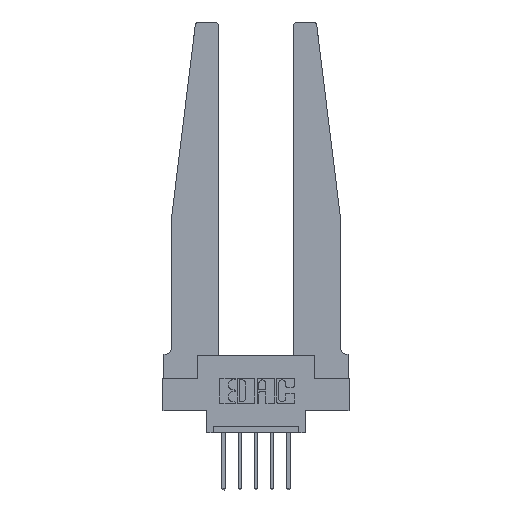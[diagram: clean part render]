
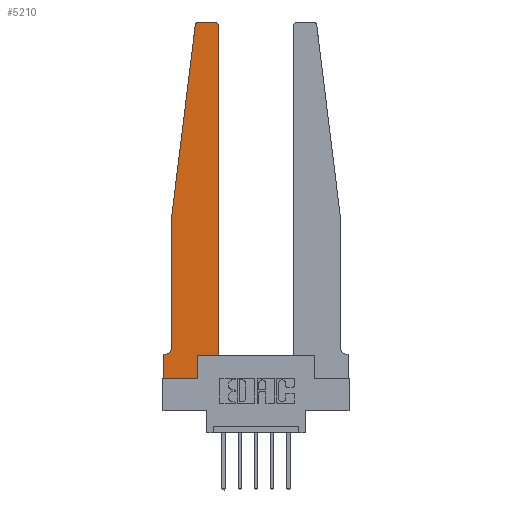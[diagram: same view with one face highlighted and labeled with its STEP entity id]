
A CAD part, top view. The second image highlights one B-rep face of the part: STEP entity #5210.
In plain terms, the highlighted planar face has unit normal (0, 0, 1).
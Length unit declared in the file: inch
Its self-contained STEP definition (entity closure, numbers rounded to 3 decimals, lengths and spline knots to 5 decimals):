
#15 = ORIENTED_EDGE ( 'NONE', *, *, #7606, .T. ) ;
#310 = CARTESIAN_POINT ( 'NONE',  ( 0., 0., 0.37 ) ) ;
#470 = CARTESIAN_POINT ( 'NONE',  ( 0.065, 1.25, 0.37 ) ) ;
#858 = ORIENTED_EDGE ( 'NONE', *, *, #10404, .T. ) ;
#1111 = VERTEX_POINT ( 'NONE', #8150 ) ;
#1137 = LINE ( 'NONE', #5262, #3582 ) ;
#1139 = LINE ( 'NONE', #310, #9951 ) ;
#1143 = ORIENTED_EDGE ( 'NONE', *, *, #5198, .T. ) ;
#1299 = VECTOR ( 'NONE', #4682, 39.37008 ) ;
#1489 = CARTESIAN_POINT ( 'NONE',  ( 0.2605, 0., 0.37 ) ) ;
#1710 = VECTOR ( 'NONE', #10399, 39.37008 ) ;
#1847 = LINE ( 'NONE', #5696, #1299 ) ;
#2155 = LINE ( 'NONE', #5459, #3050 ) ;
#2322 = CARTESIAN_POINT ( 'NONE',  ( 0.065, 0.2375, 0.37 ) ) ;
#2347 = CARTESIAN_POINT ( 'NONE',  ( 0.015, 0.1875, 0.37 ) ) ;
#2419 = DIRECTION ( 'NONE',  ( 0., 0., 1. ) ) ;
#2442 = ORIENTED_EDGE ( 'NONE', *, *, #10796, .T. ) ;
#2529 = AXIS2_PLACEMENT_3D ( 'NONE', #10632, #11456, #9399 ) ;
#2594 = DIRECTION ( 'NONE',  ( 0., 0., 1. ) ) ;
#2782 = DIRECTION ( 'NONE',  ( -0.122, -0.992, 0. ) ) ;
#2896 = EDGE_CURVE ( 'NONE', #4241, #7822, #4874, .T. ) ;
#3050 = VECTOR ( 'NONE', #6332, 39.37008 ) ;
#3070 = DIRECTION ( 'NONE',  ( -1., 0., 0. ) ) ;
#3111 = ORIENTED_EDGE ( 'NONE', *, *, #9497, .T. ) ;
#3201 = CARTESIAN_POINT ( 'NONE',  ( 0.2605, 0.18, 0.37 ) ) ;
#3289 = CARTESIAN_POINT ( 'NONE',  ( 0.27653, 2.72, 0.37 ) ) ;
#3471 = VECTOR ( 'NONE', #6698, 39.37008 ) ;
#3582 = VECTOR ( 'NONE', #6474, 39.37008 ) ;
#3888 = CARTESIAN_POINT ( 'NONE',  ( 0.24675, 2.72367, 0.37 ) ) ;
#3962 = VERTEX_POINT ( 'NONE', #2347 ) ;
#4011 = VECTOR ( 'NONE', #4735, 39.37008 ) ;
#4117 = FACE_OUTER_BOUND ( 'NONE', #6228, .T. ) ;
#4241 = VERTEX_POINT ( 'NONE', #7276 ) ;
#4321 = VERTEX_POINT ( 'NONE', #10408 ) ;
#4635 = VERTEX_POINT ( 'NONE', #3888 ) ;
#4682 = DIRECTION ( 'NONE',  ( 1., 0., 0. ) ) ;
#4735 = DIRECTION ( 'NONE',  ( 0., 1., 0. ) ) ;
#4874 = LINE ( 'NONE', #11948, #4011 ) ;
#5132 = VERTEX_POINT ( 'NONE', #6208 ) ;
#5198 = EDGE_CURVE ( 'NONE', #6388, #4241, #1137, .T. ) ;
#5210 = ADVANCED_FACE ( 'NONE', ( #4117 ), #7231, .T. ) ;
#5262 = CARTESIAN_POINT ( 'NONE',  ( 0.425, 0.18, 0.37 ) ) ;
#5318 = DIRECTION ( 'NONE',  ( 1., 0., 0. ) ) ;
#5350 = CARTESIAN_POINT ( 'NONE',  ( 0., 0., 0.37 ) ) ;
#5363 = ORIENTED_EDGE ( 'NONE', *, *, #8196, .T. ) ;
#5385 = CIRCLE ( 'NONE', #7323, 0.03 ) ;
#5412 = AXIS2_PLACEMENT_3D ( 'NONE', #6825, #12216, #13032 ) ;
#5459 = CARTESIAN_POINT ( 'NONE',  ( 0.065, 0.1875, 0.37 ) ) ;
#5696 = CARTESIAN_POINT ( 'NONE',  ( 0., 0., 0.37 ) ) ;
#5879 = ORIENTED_EDGE ( 'NONE', *, *, #2896, .T. ) ;
#6114 = LINE ( 'NONE', #3201, #1710 ) ;
#6208 = CARTESIAN_POINT ( 'NONE',  ( 0.065, 1.25, 0.37 ) ) ;
#6228 = EDGE_LOOP ( 'NONE', ( #6243, #3111, #2442, #15, #858, #10939, #7909, #12662, #5363, #1143, #5879, #10780 ) ) ;
#6240 = CARTESIAN_POINT ( 'NONE',  ( 0.25, 2.75, 0.37 ) ) ;
#6243 = ORIENTED_EDGE ( 'NONE', *, *, #7013, .T. ) ;
#6259 = CIRCLE ( 'NONE', #9524, 0.03 ) ;
#6289 = VERTEX_POINT ( 'NONE', #1489 ) ;
#6320 = VERTEX_POINT ( 'NONE', #5350 ) ;
#6332 = DIRECTION ( 'NONE',  ( -1., 0., 0. ) ) ;
#6388 = VERTEX_POINT ( 'NONE', #7157 ) ;
#6474 = DIRECTION ( 'NONE',  ( 1., 0., 0. ) ) ;
#6698 = DIRECTION ( 'NONE',  ( 0., -1., 0. ) ) ;
#6825 = CARTESIAN_POINT ( 'NONE',  ( 0.015, 0.2375, 0.37 ) ) ;
#6968 = CARTESIAN_POINT ( 'NONE',  ( 0.395, 2.75, 0.37 ) ) ;
#7013 = EDGE_CURVE ( 'NONE', #10320, #1111, #8153, .T. ) ;
#7157 = CARTESIAN_POINT ( 'NONE',  ( 0.2605, 0.18, 0.37 ) ) ;
#7231 = PLANE ( 'NONE',  #2529 ) ;
#7258 = EDGE_CURVE ( 'NONE', #6320, #6289, #1847, .T. ) ;
#7276 = CARTESIAN_POINT ( 'NONE',  ( 0.425, 0.18, 0.37 ) ) ;
#7323 = AXIS2_PLACEMENT_3D ( 'NONE', #11902, #2594, #8484 ) ;
#7368 = DIRECTION ( 'NONE',  ( 0., -1., 0. ) ) ;
#7606 = EDGE_CURVE ( 'NONE', #5132, #11706, #10921, .T. ) ;
#7822 = VERTEX_POINT ( 'NONE', #10237 ) ;
#7873 = LINE ( 'NONE', #11140, #11730 ) ;
#7909 = ORIENTED_EDGE ( 'NONE', *, *, #7954, .T. ) ;
#7954 = EDGE_CURVE ( 'NONE', #4321, #6320, #1139, .T. ) ;
#8150 = CARTESIAN_POINT ( 'NONE',  ( 0.27653, 2.75, 0.37 ) ) ;
#8153 = LINE ( 'NONE', #6240, #9737 ) ;
#8196 = EDGE_CURVE ( 'NONE', #6289, #6388, #6114, .T. ) ;
#8425 = EDGE_CURVE ( 'NONE', #7822, #10320, #5385, .T. ) ;
#8484 = DIRECTION ( 'NONE',  ( 1., 0., 0. ) ) ;
#9115 = CIRCLE ( 'NONE', #5412, 0.05 ) ;
#9399 = DIRECTION ( 'NONE',  ( 1., 0., 0. ) ) ;
#9497 = EDGE_CURVE ( 'NONE', #1111, #4635, #6259, .T. ) ;
#9524 = AXIS2_PLACEMENT_3D ( 'NONE', #3289, #2419, #5318 ) ;
#9737 = VECTOR ( 'NONE', #3070, 39.37008 ) ;
#9951 = VECTOR ( 'NONE', #7368, 39.37008 ) ;
#10237 = CARTESIAN_POINT ( 'NONE',  ( 0.425, 2.72, 0.37 ) ) ;
#10320 = VERTEX_POINT ( 'NONE', #6968 ) ;
#10399 = DIRECTION ( 'NONE',  ( 0., 1., 0. ) ) ;
#10404 = EDGE_CURVE ( 'NONE', #11706, #3962, #9115, .T. ) ;
#10408 = CARTESIAN_POINT ( 'NONE',  ( 0., 0.1875, 0.37 ) ) ;
#10632 = CARTESIAN_POINT ( 'NONE',  ( 0., 0.1875, 0.37 ) ) ;
#10780 = ORIENTED_EDGE ( 'NONE', *, *, #8425, .T. ) ;
#10796 = EDGE_CURVE ( 'NONE', #4635, #5132, #7873, .T. ) ;
#10899 = EDGE_CURVE ( 'NONE', #3962, #4321, #2155, .T. ) ;
#10921 = LINE ( 'NONE', #470, #3471 ) ;
#10939 = ORIENTED_EDGE ( 'NONE', *, *, #10899, .T. ) ;
#11140 = CARTESIAN_POINT ( 'NONE',  ( 0.065, 1.25, 0.37 ) ) ;
#11456 = DIRECTION ( 'NONE',  ( 0., 0., 1. ) ) ;
#11706 = VERTEX_POINT ( 'NONE', #2322 ) ;
#11730 = VECTOR ( 'NONE', #2782, 39.37008 ) ;
#11902 = CARTESIAN_POINT ( 'NONE',  ( 0.395, 2.72, 0.37 ) ) ;
#11948 = CARTESIAN_POINT ( 'NONE',  ( 0.425, 0.18, 0.37 ) ) ;
#12216 = DIRECTION ( 'NONE',  ( 0., 0., -1. ) ) ;
#12662 = ORIENTED_EDGE ( 'NONE', *, *, #7258, .T. ) ;
#13032 = DIRECTION ( 'NONE',  ( -1., 0., 0. ) ) ;
